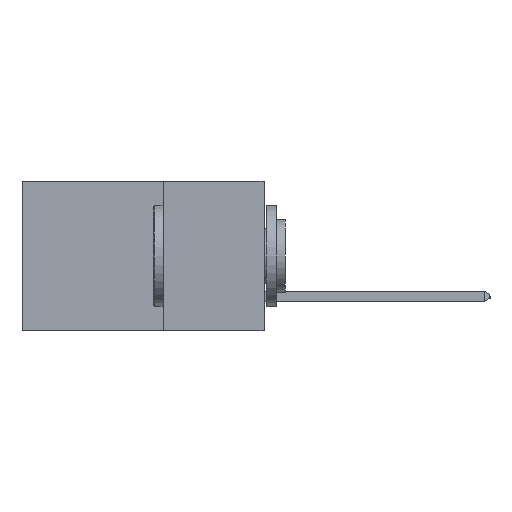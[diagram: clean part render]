
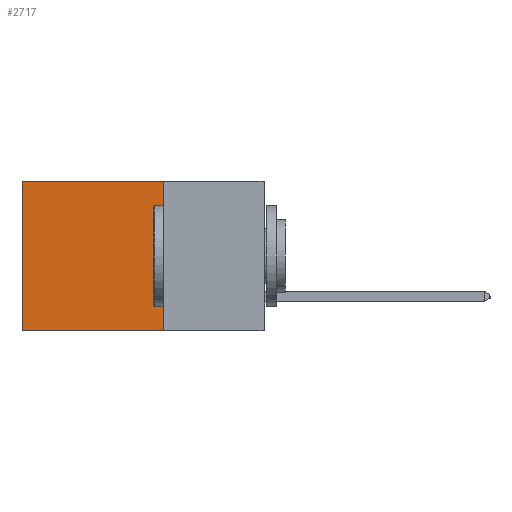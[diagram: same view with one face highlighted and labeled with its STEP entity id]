
A CAD part, left-side view. The second image highlights one B-rep face of the part: STEP entity #2717.
In plain terms, the highlighted planar face has unit normal (-1, 0, 0).
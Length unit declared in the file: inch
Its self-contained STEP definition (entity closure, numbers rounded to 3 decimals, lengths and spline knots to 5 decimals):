
#1206 = EDGE_CURVE ( 'NONE', #13493, #3878, #16466, .T. ) ;
#1897 = DIRECTION ( 'NONE',  ( 0., 0., -1. ) ) ;
#1997 = CARTESIAN_POINT ( 'NONE',  ( 0.298, 0.6, -0.37 ) ) ;
#2717 = ADVANCED_FACE ( 'NONE', ( #8059 ), #9616, .F. ) ;
#3015 = VECTOR ( 'NONE', #1897, 39.37008 ) ;
#3149 = VECTOR ( 'NONE', #11157, 39.37008 ) ;
#3607 = VECTOR ( 'NONE', #17877, 39.37008 ) ;
#3878 = VERTEX_POINT ( 'NONE', #1997 ) ;
#4022 = CARTESIAN_POINT ( 'NONE',  ( 0.298, 0.25, 0. ) ) ;
#4121 = DIRECTION ( 'NONE',  ( 1., 0., 0. ) ) ;
#4718 = CARTESIAN_POINT ( 'NONE',  ( 0.298, 0.25, 0. ) ) ;
#5194 = CARTESIAN_POINT ( 'NONE',  ( 0.298, 0.25, 0. ) ) ;
#5652 = ORIENTED_EDGE ( 'NONE', *, *, #19198, .F. ) ;
#6129 = VERTEX_POINT ( 'NONE', #20011 ) ;
#6792 = CARTESIAN_POINT ( 'NONE',  ( 0.298, 0.25, -0.37 ) ) ;
#7308 = LINE ( 'NONE', #5194, #3015 ) ;
#8059 = FACE_OUTER_BOUND ( 'NONE', #12039, .T. ) ;
#8123 = CARTESIAN_POINT ( 'NONE',  ( 0.298, 0.25, 0. ) ) ;
#8814 = ORIENTED_EDGE ( 'NONE', *, *, #20225, .T. ) ;
#9556 = CARTESIAN_POINT ( 'NONE',  ( 0.298, 0.6, 0. ) ) ;
#9616 = PLANE ( 'NONE',  #14391 ) ;
#9756 = DIRECTION ( 'NONE',  ( 0., 1., 0. ) ) ;
#10078 = LINE ( 'NONE', #8123, #18089 ) ;
#11157 = DIRECTION ( 'NONE',  ( 0., 0., -1. ) ) ;
#11721 = LINE ( 'NONE', #9556, #3149 ) ;
#12039 = EDGE_LOOP ( 'NONE', ( #20634, #14652, #5652, #8814 ) ) ;
#13493 = VERTEX_POINT ( 'NONE', #16667 ) ;
#14131 = VERTEX_POINT ( 'NONE', #4718 ) ;
#14391 = AXIS2_PLACEMENT_3D ( 'NONE', #4022, #4121, #18669 ) ;
#14652 = ORIENTED_EDGE ( 'NONE', *, *, #1206, .F. ) ;
#16466 = LINE ( 'NONE', #6792, #3607 ) ;
#16667 = CARTESIAN_POINT ( 'NONE',  ( 0.298, 0.25, -0.37 ) ) ;
#17609 = EDGE_CURVE ( 'NONE', #6129, #3878, #11721, .T. ) ;
#17877 = DIRECTION ( 'NONE',  ( 0., 1., 0. ) ) ;
#18089 = VECTOR ( 'NONE', #9756, 39.37008 ) ;
#18669 = DIRECTION ( 'NONE',  ( 0., 0., -1. ) ) ;
#19198 = EDGE_CURVE ( 'NONE', #14131, #13493, #7308, .T. ) ;
#20011 = CARTESIAN_POINT ( 'NONE',  ( 0.298, 0.6, 0. ) ) ;
#20225 = EDGE_CURVE ( 'NONE', #14131, #6129, #10078, .T. ) ;
#20634 = ORIENTED_EDGE ( 'NONE', *, *, #17609, .T. ) ;
